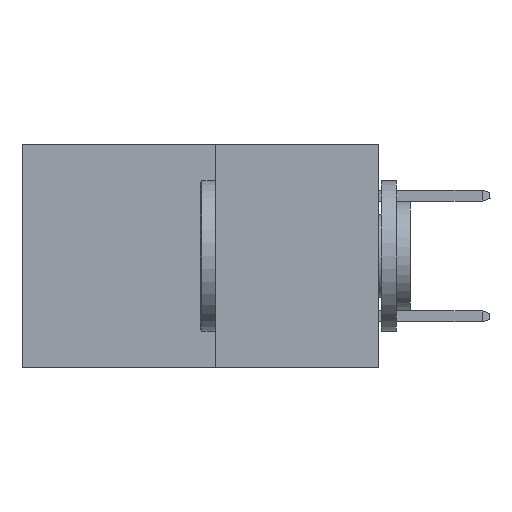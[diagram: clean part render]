
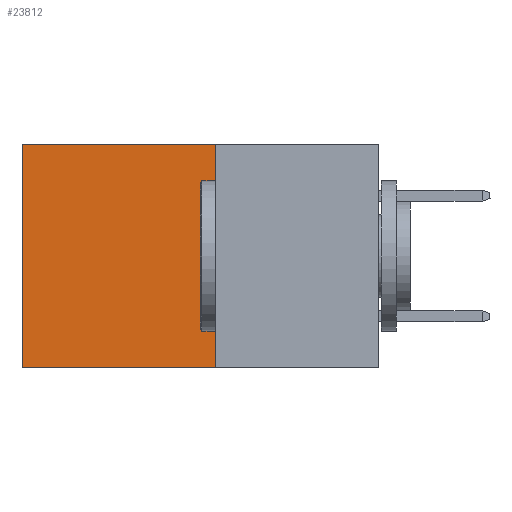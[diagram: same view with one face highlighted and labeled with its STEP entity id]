
A CAD part, left-side view. The second image highlights one B-rep face of the part: STEP entity #23812.
In plain terms, the highlighted planar face has unit normal (-1, 0, 0).
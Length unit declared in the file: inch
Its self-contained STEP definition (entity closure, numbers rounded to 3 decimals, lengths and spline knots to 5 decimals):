
#872 = AXIS2_PLACEMENT_3D ( 'NONE', #895, #14520, #2837 ) ;
#895 = CARTESIAN_POINT ( 'NONE',  ( 0.277, 0.27, -0.37 ) ) ;
#1621 = CARTESIAN_POINT ( 'NONE',  ( 0.277, 0.27, -0.37 ) ) ;
#1852 = VERTEX_POINT ( 'NONE', #5468 ) ;
#2305 = VECTOR ( 'NONE', #3580, 39.37008 ) ;
#2837 = DIRECTION ( 'NONE',  ( 0., 0., -1. ) ) ;
#2964 = CARTESIAN_POINT ( 'NONE',  ( 0.277, 0.27, 0. ) ) ;
#3580 = DIRECTION ( 'NONE',  ( 0., 1., 0. ) ) ;
#4439 = ORIENTED_EDGE ( 'NONE', *, *, #12561, .F. ) ;
#4825 = ORIENTED_EDGE ( 'NONE', *, *, #13324, .T. ) ;
#5468 = CARTESIAN_POINT ( 'NONE',  ( 0.277, 0.59, 0. ) ) ;
#5807 = EDGE_CURVE ( 'NONE', #1852, #8304, #17534, .T. ) ;
#6098 = CARTESIAN_POINT ( 'NONE',  ( 0.277, 0.27, -0.37 ) ) ;
#7104 = VERTEX_POINT ( 'NONE', #7271 ) ;
#7271 = CARTESIAN_POINT ( 'NONE',  ( 0.277, 0.27, -0.37 ) ) ;
#7516 = LINE ( 'NONE', #1621, #2305 ) ;
#8097 = DIRECTION ( 'NONE',  ( 0., 0., -1. ) ) ;
#8304 = VERTEX_POINT ( 'NONE', #14375 ) ;
#8568 = ORIENTED_EDGE ( 'NONE', *, *, #5807, .T. ) ;
#9251 = CARTESIAN_POINT ( 'NONE',  ( 0.277, 0.59, -0.37 ) ) ;
#9422 = DIRECTION ( 'NONE',  ( 0., 0., -1. ) ) ;
#10310 = EDGE_CURVE ( 'NONE', #7104, #8304, #7516, .T. ) ;
#12561 = EDGE_CURVE ( 'NONE', #12860, #7104, #13533, .T. ) ;
#12570 = PLANE ( 'NONE',  #872 ) ;
#12860 = VERTEX_POINT ( 'NONE', #12925 ) ;
#12925 = CARTESIAN_POINT ( 'NONE',  ( 0.277, 0.27, 0. ) ) ;
#13138 = FACE_OUTER_BOUND ( 'NONE', #19595, .T. ) ;
#13324 = EDGE_CURVE ( 'NONE', #12860, #1852, #14861, .T. ) ;
#13533 = LINE ( 'NONE', #6098, #23181 ) ;
#14375 = CARTESIAN_POINT ( 'NONE',  ( 0.277, 0.59, -0.37 ) ) ;
#14520 = DIRECTION ( 'NONE',  ( 1., 0., 0. ) ) ;
#14861 = LINE ( 'NONE', #2964, #24462 ) ;
#16609 = DIRECTION ( 'NONE',  ( 0., 1., 0. ) ) ;
#16753 = ORIENTED_EDGE ( 'NONE', *, *, #10310, .F. ) ;
#17534 = LINE ( 'NONE', #9251, #21439 ) ;
#19595 = EDGE_LOOP ( 'NONE', ( #8568, #16753, #4439, #4825 ) ) ;
#21439 = VECTOR ( 'NONE', #9422, 39.37008 ) ;
#23181 = VECTOR ( 'NONE', #8097, 39.37008 ) ;
#23812 = ADVANCED_FACE ( 'NONE', ( #13138 ), #12570, .F. ) ;
#24462 = VECTOR ( 'NONE', #16609, 39.37008 ) ;
